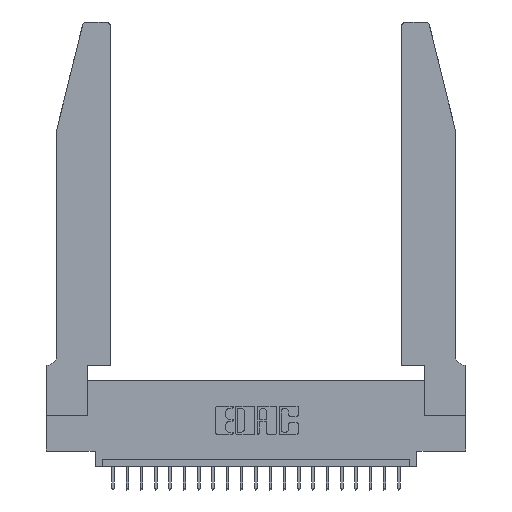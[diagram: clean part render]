
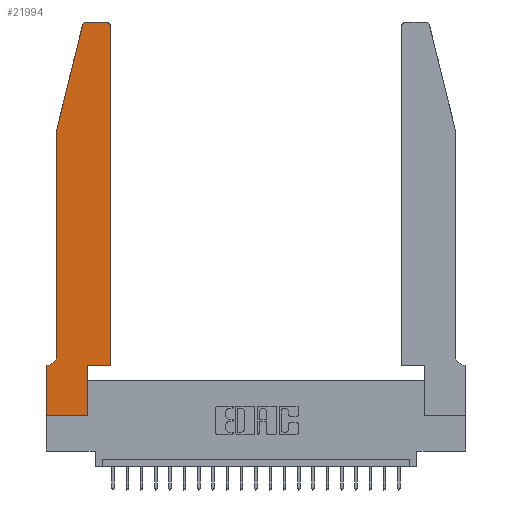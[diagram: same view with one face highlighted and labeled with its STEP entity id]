
A CAD part, top view. The second image highlights one B-rep face of the part: STEP entity #21994.
In plain terms, the highlighted planar face has unit normal (0, 0, 1).
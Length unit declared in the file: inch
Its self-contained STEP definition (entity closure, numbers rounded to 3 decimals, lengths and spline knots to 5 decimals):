
#82 = DIRECTION ( 'NONE',  ( 0., -1., 0. ) ) ;
#239 = VECTOR ( 'NONE', #82, 39.37008 ) ;
#389 = DIRECTION ( 'NONE',  ( 1., 0., 0. ) ) ;
#496 = VERTEX_POINT ( 'NONE', #7933 ) ;
#624 = EDGE_CURVE ( 'NONE', #19001, #4589, #4395, .T. ) ;
#1684 = FACE_OUTER_BOUND ( 'NONE', #16289, .T. ) ;
#1824 = VERTEX_POINT ( 'NONE', #4137 ) ;
#2180 = DIRECTION ( 'NONE',  ( 1., 0., 0. ) ) ;
#2654 = CARTESIAN_POINT ( 'NONE',  ( 0.25487, 2.72718, 0.37 ) ) ;
#2737 = CARTESIAN_POINT ( 'NONE',  ( 0.2865, 0.35, 0.37 ) ) ;
#2774 = CARTESIAN_POINT ( 'NONE',  ( 0.2865, 0.35, 0.37 ) ) ;
#3081 = VECTOR ( 'NONE', #22317, 39.37008 ) ;
#3250 = DIRECTION ( 'NONE',  ( 1., 0., 0. ) ) ;
#3317 = ORIENTED_EDGE ( 'NONE', *, *, #624, .T. ) ;
#3680 = LINE ( 'NONE', #9425, #3081 ) ;
#3689 = ORIENTED_EDGE ( 'NONE', *, *, #21515, .T. ) ;
#3757 = DIRECTION ( 'NONE',  ( 0., 0., 1. ) ) ;
#4137 = CARTESIAN_POINT ( 'NONE',  ( 0., 0., 0.37 ) ) ;
#4395 = LINE ( 'NONE', #2774, #13212 ) ;
#4589 = VERTEX_POINT ( 'NONE', #2737 ) ;
#4708 = AXIS2_PLACEMENT_3D ( 'NONE', #22106, #22272, #2180 ) ;
#5344 = EDGE_CURVE ( 'NONE', #4589, #13771, #14734, .T. ) ;
#5931 = CARTESIAN_POINT ( 'NONE',  ( 0., 0.35, 0.37 ) ) ;
#6153 = DIRECTION ( 'NONE',  ( -1., 0., 0. ) ) ;
#6311 = CARTESIAN_POINT ( 'NONE',  ( 0.0055, 0.42, 0.37 ) ) ;
#6313 = AXIS2_PLACEMENT_3D ( 'NONE', #6311, #11614, #8034 ) ;
#7088 = CARTESIAN_POINT ( 'NONE',  ( 0.4505, 0.35, 0.37 ) ) ;
#7091 = EDGE_CURVE ( 'NONE', #17208, #19910, #11828, .T. ) ;
#7372 = EDGE_CURVE ( 'NONE', #19910, #11690, #13507, .T. ) ;
#7543 = EDGE_CURVE ( 'NONE', #14963, #1824, #8396, .T. ) ;
#7933 = CARTESIAN_POINT ( 'NONE',  ( 0.0055, 0.35, 0.37 ) ) ;
#7934 = DIRECTION ( 'NONE',  ( 1., 0., 0. ) ) ;
#8034 = DIRECTION ( 'NONE',  ( -1., 0., 0. ) ) ;
#8153 = DIRECTION ( 'NONE',  ( 1., 0., 0. ) ) ;
#8396 = LINE ( 'NONE', #15913, #17740 ) ;
#8713 = EDGE_CURVE ( 'NONE', #1824, #19001, #15629, .T. ) ;
#8907 = CARTESIAN_POINT ( 'NONE',  ( 0.0755, 2., 0.37 ) ) ;
#9341 = CARTESIAN_POINT ( 'NONE',  ( 0.0755, 2., 0.37 ) ) ;
#9425 = CARTESIAN_POINT ( 'NONE',  ( 0.0755, 2., 0.37 ) ) ;
#9617 = PLANE ( 'NONE',  #4708 ) ;
#9726 = CARTESIAN_POINT ( 'NONE',  ( 0.0755, 0.35, 0.37 ) ) ;
#9967 = CIRCLE ( 'NONE', #6313, 0.07 ) ;
#10324 = CARTESIAN_POINT ( 'NONE',  ( 0., 0., 0.37 ) ) ;
#10428 = CIRCLE ( 'NONE', #21684, 0.03 ) ;
#10486 = EDGE_CURVE ( 'NONE', #14839, #17208, #10428, .T. ) ;
#10510 = VECTOR ( 'NONE', #7934, 39.37008 ) ;
#10564 = CARTESIAN_POINT ( 'NONE',  ( 0.284, 2.75, 0.37 ) ) ;
#10732 = DIRECTION ( 'NONE',  ( -1., 0., 0. ) ) ;
#10803 = VECTOR ( 'NONE', #3250, 39.37008 ) ;
#11377 = CARTESIAN_POINT ( 'NONE',  ( 0.4205, 2.75, 0.37 ) ) ;
#11614 = DIRECTION ( 'NONE',  ( 0., 0., -1. ) ) ;
#11690 = VERTEX_POINT ( 'NONE', #2654 ) ;
#11828 = LINE ( 'NONE', #17932, #20929 ) ;
#12397 = DIRECTION ( 'NONE',  ( 0., -1., 0. ) ) ;
#12573 = ORIENTED_EDGE ( 'NONE', *, *, #7091, .T. ) ;
#13212 = VECTOR ( 'NONE', #13557, 39.37008 ) ;
#13507 = CIRCLE ( 'NONE', #18108, 0.03 ) ;
#13557 = DIRECTION ( 'NONE',  ( 0., 1., 0. ) ) ;
#13771 = VERTEX_POINT ( 'NONE', #7088 ) ;
#14274 = ORIENTED_EDGE ( 'NONE', *, *, #5344, .T. ) ;
#14675 = CARTESIAN_POINT ( 'NONE',  ( 0.4205, 2.72, 0.37 ) ) ;
#14734 = LINE ( 'NONE', #22642, #10510 ) ;
#14839 = VERTEX_POINT ( 'NONE', #22778 ) ;
#14963 = VERTEX_POINT ( 'NONE', #5931 ) ;
#15561 = CARTESIAN_POINT ( 'NONE',  ( 0.0755, 0.42, 0.37 ) ) ;
#15629 = LINE ( 'NONE', #10324, #10803 ) ;
#15707 = VERTEX_POINT ( 'NONE', #8907 ) ;
#15889 = VECTOR ( 'NONE', #23323, 39.37008 ) ;
#15913 = CARTESIAN_POINT ( 'NONE',  ( 0., 0., 0.37 ) ) ;
#16156 = LINE ( 'NONE', #19499, #15889 ) ;
#16289 = EDGE_LOOP ( 'NONE', ( #12573, #20095, #17395, #23388, #22423, #3689, #21205, #20493, #3317, #14274, #18132, #17981 ) ) ;
#17208 = VERTEX_POINT ( 'NONE', #11377 ) ;
#17395 = ORIENTED_EDGE ( 'NONE', *, *, #22750, .T. ) ;
#17740 = VECTOR ( 'NONE', #12397, 39.37008 ) ;
#17750 = CARTESIAN_POINT ( 'NONE',  ( 0.2865, 0., 0.37 ) ) ;
#17932 = CARTESIAN_POINT ( 'NONE',  ( 0.2605, 2.75, 0.37 ) ) ;
#17981 = ORIENTED_EDGE ( 'NONE', *, *, #10486, .T. ) ;
#18108 = AXIS2_PLACEMENT_3D ( 'NONE', #19335, #22885, #8153 ) ;
#18132 = ORIENTED_EDGE ( 'NONE', *, *, #22539, .T. ) ;
#18490 = LINE ( 'NONE', #9726, #21326 ) ;
#19001 = VERTEX_POINT ( 'NONE', #17750 ) ;
#19335 = CARTESIAN_POINT ( 'NONE',  ( 0.284, 2.72, 0.37 ) ) ;
#19499 = CARTESIAN_POINT ( 'NONE',  ( 0.4505, 0.35, 0.37 ) ) ;
#19910 = VERTEX_POINT ( 'NONE', #10564 ) ;
#20095 = ORIENTED_EDGE ( 'NONE', *, *, #7372, .T. ) ;
#20493 = ORIENTED_EDGE ( 'NONE', *, *, #8713, .T. ) ;
#20740 = EDGE_CURVE ( 'NONE', #15707, #22330, #23283, .T. ) ;
#20929 = VECTOR ( 'NONE', #10732, 39.37008 ) ;
#21205 = ORIENTED_EDGE ( 'NONE', *, *, #7543, .T. ) ;
#21326 = VECTOR ( 'NONE', #6153, 39.37008 ) ;
#21415 = EDGE_CURVE ( 'NONE', #22330, #496, #9967, .T. ) ;
#21515 = EDGE_CURVE ( 'NONE', #496, #14963, #18490, .T. ) ;
#21684 = AXIS2_PLACEMENT_3D ( 'NONE', #14675, #3757, #389 ) ;
#21994 = ADVANCED_FACE ( 'NONE', ( #1684 ), #9617, .T. ) ;
#22106 = CARTESIAN_POINT ( 'NONE',  ( 0., 0.35, 0.37 ) ) ;
#22272 = DIRECTION ( 'NONE',  ( 0., 0., 1. ) ) ;
#22317 = DIRECTION ( 'NONE',  ( -0.239, -0.971, 0. ) ) ;
#22330 = VERTEX_POINT ( 'NONE', #15561 ) ;
#22423 = ORIENTED_EDGE ( 'NONE', *, *, #21415, .T. ) ;
#22539 = EDGE_CURVE ( 'NONE', #13771, #14839, #16156, .T. ) ;
#22642 = CARTESIAN_POINT ( 'NONE',  ( 0.4505, 0.35, 0.37 ) ) ;
#22750 = EDGE_CURVE ( 'NONE', #11690, #15707, #3680, .T. ) ;
#22778 = CARTESIAN_POINT ( 'NONE',  ( 0.4505, 2.72, 0.37 ) ) ;
#22885 = DIRECTION ( 'NONE',  ( 0., 0., 1. ) ) ;
#23283 = LINE ( 'NONE', #9341, #239 ) ;
#23323 = DIRECTION ( 'NONE',  ( 0., 1., 0. ) ) ;
#23388 = ORIENTED_EDGE ( 'NONE', *, *, #20740, .T. ) ;
